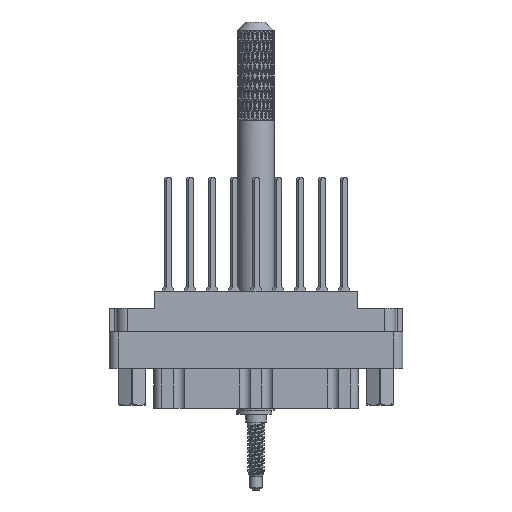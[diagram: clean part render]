
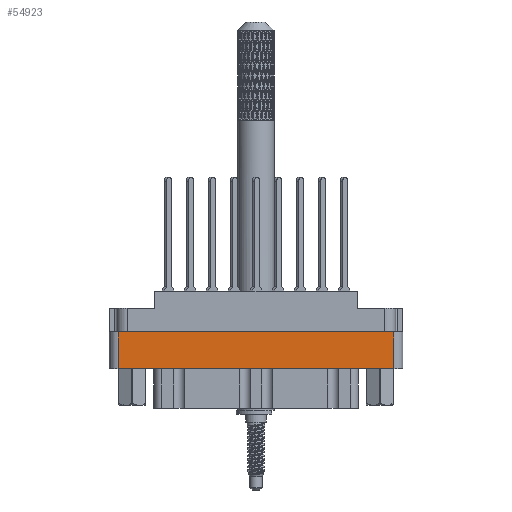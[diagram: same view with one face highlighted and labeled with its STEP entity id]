
A CAD part, front view. The second image highlights one B-rep face of the part: STEP entity #54923.
In plain terms, the highlighted planar face has unit normal (0, -1, 0).
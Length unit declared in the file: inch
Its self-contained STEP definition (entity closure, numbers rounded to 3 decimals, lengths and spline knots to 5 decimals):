
#601 = LINE ( 'NONE', #94225, #82918 ) ;
#2301 = VECTOR ( 'NONE', #102959, 39.37008 ) ;
#4264 = EDGE_CURVE ( 'NONE', #42646, #84665, #30020, .T. ) ;
#4319 = EDGE_CURVE ( 'NONE', #102358, #42646, #21596, .T. ) ;
#10122 = FACE_OUTER_BOUND ( 'NONE', #52533, .T. ) ;
#10919 = DIRECTION ( 'NONE',  ( 1., 0., 0. ) ) ;
#13559 = VECTOR ( 'NONE', #45667, 39.37008 ) ;
#19195 = CARTESIAN_POINT ( 'NONE',  ( -0.938, -0.438, -0.529 ) ) ;
#20756 = CARTESIAN_POINT ( 'NONE',  ( 0.938, -0.438, -0.529 ) ) ;
#21040 = CARTESIAN_POINT ( 'NONE',  ( -0.938, -0.438, -0.798 ) ) ;
#21596 = LINE ( 'NONE', #21040, #13559 ) ;
#23799 = EDGE_CURVE ( 'NONE', #67679, #102358, #601, .T. ) ;
#30020 = LINE ( 'NONE', #61960, #72634 ) ;
#34783 = PLANE ( 'NONE',  #108723 ) ;
#35892 = ORIENTED_EDGE ( 'NONE', *, *, #57914, .T. ) ;
#37407 = ORIENTED_EDGE ( 'NONE', *, *, #4264, .F. ) ;
#41555 = CARTESIAN_POINT ( 'NONE',  ( 0.938, -0.438, -0.277 ) ) ;
#42646 = VERTEX_POINT ( 'NONE', #58033 ) ;
#44321 = DIRECTION ( 'NONE',  ( 0., 0., -1. ) ) ;
#45667 = DIRECTION ( 'NONE',  ( 0., 0., 1. ) ) ;
#50820 = CARTESIAN_POINT ( 'NONE',  ( 0.938, -0.438, -0.798 ) ) ;
#52533 = EDGE_LOOP ( 'NONE', ( #94902, #79538, #35892, #37407 ) ) ;
#54923 = ADVANCED_FACE ( 'NONE', ( #10122 ), #34783, .T. ) ;
#57914 = EDGE_CURVE ( 'NONE', #67679, #84665, #86118, .T. ) ;
#58033 = CARTESIAN_POINT ( 'NONE',  ( -0.938, -0.438, -0.277 ) ) ;
#61960 = CARTESIAN_POINT ( 'NONE',  ( -1., -0.438, -0.277 ) ) ;
#67679 = VERTEX_POINT ( 'NONE', #20756 ) ;
#72634 = VECTOR ( 'NONE', #10919, 39.37008 ) ;
#77378 = DIRECTION ( 'NONE',  ( -1., 0., 0. ) ) ;
#79538 = ORIENTED_EDGE ( 'NONE', *, *, #23799, .F. ) ;
#82918 = VECTOR ( 'NONE', #77378, 39.37008 ) ;
#84665 = VERTEX_POINT ( 'NONE', #41555 ) ;
#86118 = LINE ( 'NONE', #50820, #2301 ) ;
#94225 = CARTESIAN_POINT ( 'NONE',  ( 0.938, -0.438, -0.529 ) ) ;
#94902 = ORIENTED_EDGE ( 'NONE', *, *, #4319, .F. ) ;
#95325 = DIRECTION ( 'NONE',  ( 0., -1., 0. ) ) ;
#102358 = VERTEX_POINT ( 'NONE', #19195 ) ;
#102959 = DIRECTION ( 'NONE',  ( 0., 0., 1. ) ) ;
#103761 = CARTESIAN_POINT ( 'NONE',  ( -0.938, -0.438, -0.798 ) ) ;
#108723 = AXIS2_PLACEMENT_3D ( 'NONE', #103761, #95325, #44321 ) ;
